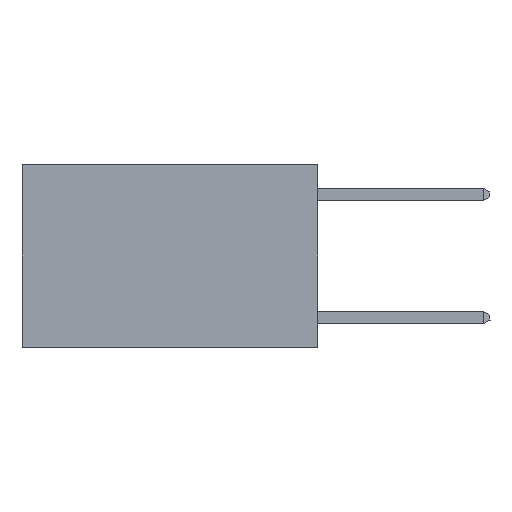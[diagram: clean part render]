
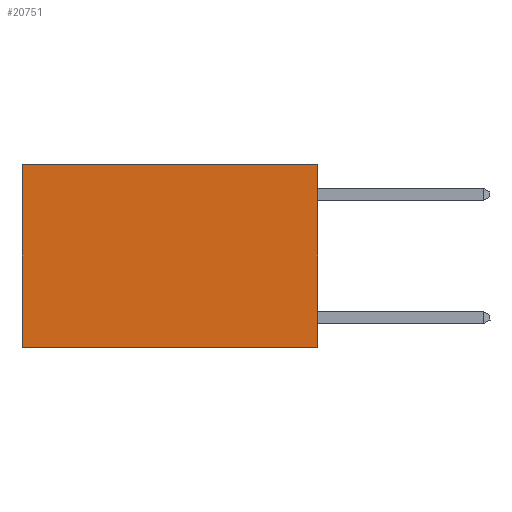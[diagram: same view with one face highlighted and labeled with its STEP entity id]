
A CAD part, left-side view. The second image highlights one B-rep face of the part: STEP entity #20751.
In plain terms, the highlighted planar face has unit normal (-1, 0, 0).
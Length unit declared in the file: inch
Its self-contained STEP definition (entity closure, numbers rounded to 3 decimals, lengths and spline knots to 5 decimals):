
#20 = EDGE_LOOP ( 'NONE', ( #752, #889, #1050, #1098 ) ) ;
#752 = ORIENTED_EDGE ( 'NONE', *, *, #22420, .T. ) ;
#889 = ORIENTED_EDGE ( 'NONE', *, *, #5417, .F. ) ;
#1050 = ORIENTED_EDGE ( 'NONE', *, *, #20760, .F. ) ;
#1098 = ORIENTED_EDGE ( 'NONE', *, *, #2292, .T. ) ;
#2292 = EDGE_CURVE ( 'NONE', #5418, #22047, #2717, .T. ) ;
#2371 = VECTOR ( 'NONE', #14476, 39.37008 ) ;
#2717 = LINE ( 'NONE', #12402, #20833 ) ;
#2955 = CARTESIAN_POINT ( 'NONE',  ( 0.2625, 0., 0. ) ) ;
#3224 = LINE ( 'NONE', #17729, #17561 ) ;
#4827 = CARTESIAN_POINT ( 'NONE',  ( 0.2625, 0.6, -0.37 ) ) ;
#4830 = LINE ( 'NONE', #10535, #12485 ) ;
#5107 = PLANE ( 'NONE',  #23611 ) ;
#5417 = EDGE_CURVE ( 'NONE', #17343, #11118, #4830, .T. ) ;
#5418 = VERTEX_POINT ( 'NONE', #2955 ) ;
#8882 = DIRECTION ( 'NONE',  ( 1., 0., 0. ) ) ;
#9338 = CARTESIAN_POINT ( 'NONE',  ( 0.2625, 0.6, 0. ) ) ;
#10535 = CARTESIAN_POINT ( 'NONE',  ( 0.2625, 0., -0.37 ) ) ;
#11118 = VERTEX_POINT ( 'NONE', #4827 ) ;
#12402 = CARTESIAN_POINT ( 'NONE',  ( 0.2625, 0., 0. ) ) ;
#12485 = VECTOR ( 'NONE', #16070, 39.37008 ) ;
#12487 = LINE ( 'NONE', #23509, #2371 ) ;
#14476 = DIRECTION ( 'NONE',  ( 0., 0., -1. ) ) ;
#16070 = DIRECTION ( 'NONE',  ( 0., 1., 0. ) ) ;
#17343 = VERTEX_POINT ( 'NONE', #19136 ) ;
#17347 = FACE_OUTER_BOUND ( 'NONE', #20, .T. ) ;
#17561 = VECTOR ( 'NONE', #21384, 39.37008 ) ;
#17729 = CARTESIAN_POINT ( 'NONE',  ( 0.2625, 0.6, 0. ) ) ;
#19136 = CARTESIAN_POINT ( 'NONE',  ( 0.2625, 0., -0.37 ) ) ;
#19933 = CARTESIAN_POINT ( 'NONE',  ( 0.2625, 0., 0. ) ) ;
#20187 = DIRECTION ( 'NONE',  ( 0., 1., 0. ) ) ;
#20751 = ADVANCED_FACE ( 'NONE', ( #17347 ), #5107, .F. ) ;
#20760 = EDGE_CURVE ( 'NONE', #5418, #17343, #12487, .T. ) ;
#20833 = VECTOR ( 'NONE', #20187, 39.37008 ) ;
#21384 = DIRECTION ( 'NONE',  ( 0., 0., -1. ) ) ;
#21755 = DIRECTION ( 'NONE',  ( 0., 0., -1. ) ) ;
#22047 = VERTEX_POINT ( 'NONE', #9338 ) ;
#22420 = EDGE_CURVE ( 'NONE', #22047, #11118, #3224, .T. ) ;
#23509 = CARTESIAN_POINT ( 'NONE',  ( 0.2625, 0., 0. ) ) ;
#23611 = AXIS2_PLACEMENT_3D ( 'NONE', #19933, #8882, #21755 ) ;
